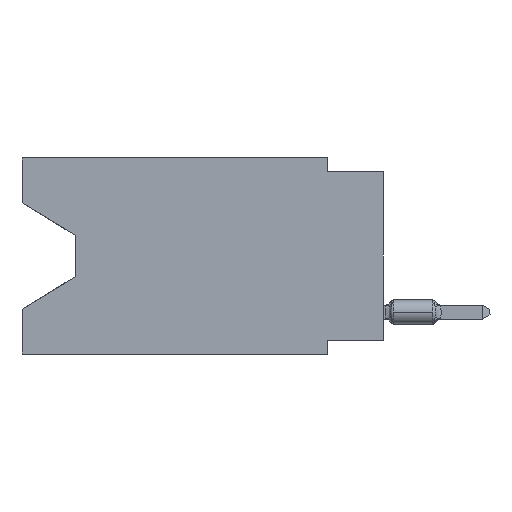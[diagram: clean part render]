
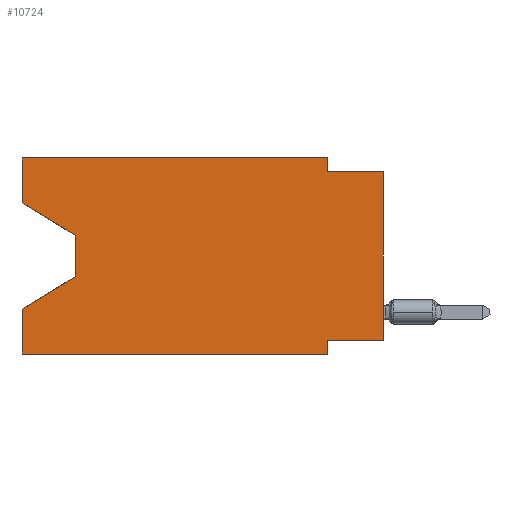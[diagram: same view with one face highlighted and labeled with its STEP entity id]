
A CAD part, left-side view. The second image highlights one B-rep face of the part: STEP entity #10724.
In plain terms, the highlighted planar face has unit normal (-1, 0, 0).
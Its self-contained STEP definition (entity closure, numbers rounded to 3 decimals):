
#278 = VERTEX_POINT ( 'NONE', #18204 ) ;
#285 = FACE_OUTER_BOUND ( 'NONE', #13902, .T. ) ;
#400 = DIRECTION ( 'NONE',  ( 0., 0., 1. ) ) ;
#1129 = CARTESIAN_POINT ( 'NONE',  ( 0., 16.383, 0. ) ) ;
#1442 = EDGE_CURVE ( 'NONE', #11655, #9051, #14736, .T. ) ;
#1532 = VECTOR ( 'NONE', #20490, 1000. ) ;
#1934 = EDGE_CURVE ( 'NONE', #10550, #17345, #22186, .T. ) ;
#1943 = DIRECTION ( 'NONE',  ( 0., 0.855, -0.519 ) ) ;
#2393 = VECTOR ( 'NONE', #400, 1000. ) ;
#2554 = CARTESIAN_POINT ( 'NONE',  ( 0., 16.383, 0. ) ) ;
#2803 = CARTESIAN_POINT ( 'NONE',  ( 0., 16.383, -6.852 ) ) ;
#2872 = VERTEX_POINT ( 'NONE', #6069 ) ;
#3043 = VECTOR ( 'NONE', #10636, 1000. ) ;
#3242 = CARTESIAN_POINT ( 'NONE',  ( 0., 0., -0.635 ) ) ;
#3255 = CARTESIAN_POINT ( 'NONE',  ( 0., 2.54, 0. ) ) ;
#3659 = VECTOR ( 'NONE', #7318, 1000. ) ;
#5485 = DIRECTION ( 'NONE',  ( 0., 0., 1. ) ) ;
#6039 = CARTESIAN_POINT ( 'NONE',  ( 0., 13.97, -3.505 ) ) ;
#6069 = CARTESIAN_POINT ( 'NONE',  ( 0., 2.54, -8.89 ) ) ;
#6123 = LINE ( 'NONE', #11718, #23180 ) ;
#6682 = ORIENTED_EDGE ( 'NONE', *, *, #22969, .T. ) ;
#6735 = EDGE_CURVE ( 'NONE', #21337, #13340, #6123, .T. ) ;
#6909 = DIRECTION ( 'NONE',  ( 0., 0., -1. ) ) ;
#6981 = VECTOR ( 'NONE', #10185, 1000. ) ;
#7128 = DIRECTION ( 'NONE',  ( 0., 0., -1. ) ) ;
#7311 = CARTESIAN_POINT ( 'NONE',  ( 0., 16.383, -8.89 ) ) ;
#7318 = DIRECTION ( 'NONE',  ( 0., 0., -1. ) ) ;
#7470 = ORIENTED_EDGE ( 'NONE', *, *, #23460, .T. ) ;
#7527 = ORIENTED_EDGE ( 'NONE', *, *, #23767, .F. ) ;
#7595 = CARTESIAN_POINT ( 'NONE',  ( 0., 0., -0.635 ) ) ;
#7633 = EDGE_CURVE ( 'NONE', #9051, #19274, #9090, .T. ) ;
#8300 = ORIENTED_EDGE ( 'NONE', *, *, #19170, .F. ) ;
#8531 = LINE ( 'NONE', #1129, #10843 ) ;
#8708 = PLANE ( 'NONE',  #21011 ) ;
#8941 = VERTEX_POINT ( 'NONE', #7311 ) ;
#9051 = VERTEX_POINT ( 'NONE', #17484 ) ;
#9090 = LINE ( 'NONE', #23857, #21678 ) ;
#9175 = LINE ( 'NONE', #3255, #17801 ) ;
#9290 = ORIENTED_EDGE ( 'NONE', *, *, #1442, .T. ) ;
#9470 = LINE ( 'NONE', #11769, #1532 ) ;
#9491 = ORIENTED_EDGE ( 'NONE', *, *, #6735, .T. ) ;
#9552 = EDGE_CURVE ( 'NONE', #278, #13340, #19838, .T. ) ;
#9705 = ORIENTED_EDGE ( 'NONE', *, *, #9552, .F. ) ;
#9934 = LINE ( 'NONE', #11522, #6981 ) ;
#10018 = CARTESIAN_POINT ( 'NONE',  ( 0., 0., -8.255 ) ) ;
#10185 = DIRECTION ( 'NONE',  ( 0., 1., 0. ) ) ;
#10550 = VERTEX_POINT ( 'NONE', #21404 ) ;
#10609 = VERTEX_POINT ( 'NONE', #13924 ) ;
#10636 = DIRECTION ( 'NONE',  ( 0., -1., 0. ) ) ;
#10724 = ADVANCED_FACE ( 'NONE', ( #285 ), #8708, .F. ) ;
#10843 = VECTOR ( 'NONE', #21464, 1000. ) ;
#10988 = ORIENTED_EDGE ( 'NONE', *, *, #11925, .F. ) ;
#11087 = LINE ( 'NONE', #22215, #18148 ) ;
#11203 = CARTESIAN_POINT ( 'NONE',  ( 0., 13.97, -3.505 ) ) ;
#11426 = LINE ( 'NONE', #2554, #2393 ) ;
#11522 = CARTESIAN_POINT ( 'NONE',  ( 0., 0., -8.255 ) ) ;
#11655 = VERTEX_POINT ( 'NONE', #6039 ) ;
#11718 = CARTESIAN_POINT ( 'NONE',  ( 0., 0., 0. ) ) ;
#11769 = CARTESIAN_POINT ( 'NONE',  ( 0., 16.383, -2.038 ) ) ;
#11925 = EDGE_CURVE ( 'NONE', #10609, #278, #9175, .T. ) ;
#12100 = ORIENTED_EDGE ( 'NONE', *, *, #17191, .F. ) ;
#12611 = LINE ( 'NONE', #12855, #16618 ) ;
#12855 = CARTESIAN_POINT ( 'NONE',  ( 0., 2.54, -8.89 ) ) ;
#12881 = CARTESIAN_POINT ( 'NONE',  ( 0., 16.383, 0. ) ) ;
#13073 = CARTESIAN_POINT ( 'NONE',  ( 0., 16.383, 0. ) ) ;
#13144 = CARTESIAN_POINT ( 'NONE',  ( 0., 16.383, 0. ) ) ;
#13340 = VERTEX_POINT ( 'NONE', #7595 ) ;
#13426 = ORIENTED_EDGE ( 'NONE', *, *, #1934, .F. ) ;
#13751 = VECTOR ( 'NONE', #5485, 1000. ) ;
#13902 = EDGE_LOOP ( 'NONE', ( #7470, #9290, #15675, #8300, #6682, #7527, #21201, #9491, #9705, #10988, #12100, #13426 ) ) ;
#13924 = CARTESIAN_POINT ( 'NONE',  ( 0., 2.54, 0. ) ) ;
#14004 = VERTEX_POINT ( 'NONE', #19032 ) ;
#14736 = LINE ( 'NONE', #11203, #3659 ) ;
#15092 = DIRECTION ( 'NONE',  ( 1., 0., 0. ) ) ;
#15675 = ORIENTED_EDGE ( 'NONE', *, *, #7633, .T. ) ;
#15801 = EDGE_CURVE ( 'NONE', #21337, #14004, #9934, .T. ) ;
#16618 = VECTOR ( 'NONE', #6909, 1000. ) ;
#17191 = EDGE_CURVE ( 'NONE', #17345, #10609, #8531, .T. ) ;
#17345 = VERTEX_POINT ( 'NONE', #13073 ) ;
#17484 = CARTESIAN_POINT ( 'NONE',  ( 0., 13.97, -5.385 ) ) ;
#17801 = VECTOR ( 'NONE', #7128, 1000. ) ;
#18148 = VECTOR ( 'NONE', #18468, 1000. ) ;
#18204 = CARTESIAN_POINT ( 'NONE',  ( 0., 2.54, -0.635 ) ) ;
#18468 = DIRECTION ( 'NONE',  ( 0., -1., 0. ) ) ;
#19032 = CARTESIAN_POINT ( 'NONE',  ( 0., 2.54, -8.255 ) ) ;
#19091 = DIRECTION ( 'NONE',  ( 0., 0., 1. ) ) ;
#19170 = EDGE_CURVE ( 'NONE', #8941, #19274, #11426, .T. ) ;
#19274 = VERTEX_POINT ( 'NONE', #2803 ) ;
#19838 = LINE ( 'NONE', #3242, #3043 ) ;
#20490 = DIRECTION ( 'NONE',  ( 0., -0.855, -0.519 ) ) ;
#21011 = AXIS2_PLACEMENT_3D ( 'NONE', #13144, #15092, #21648 ) ;
#21201 = ORIENTED_EDGE ( 'NONE', *, *, #15801, .F. ) ;
#21337 = VERTEX_POINT ( 'NONE', #10018 ) ;
#21404 = CARTESIAN_POINT ( 'NONE',  ( 0., 16.383, -2.038 ) ) ;
#21464 = DIRECTION ( 'NONE',  ( 0., -1., 0. ) ) ;
#21648 = DIRECTION ( 'NONE',  ( 0., 0., -1. ) ) ;
#21678 = VECTOR ( 'NONE', #1943, 1000. ) ;
#22186 = LINE ( 'NONE', #12881, #13751 ) ;
#22215 = CARTESIAN_POINT ( 'NONE',  ( 0., 16.383, -8.89 ) ) ;
#22969 = EDGE_CURVE ( 'NONE', #8941, #2872, #11087, .T. ) ;
#23180 = VECTOR ( 'NONE', #19091, 1000. ) ;
#23460 = EDGE_CURVE ( 'NONE', #10550, #11655, #9470, .T. ) ;
#23767 = EDGE_CURVE ( 'NONE', #14004, #2872, #12611, .T. ) ;
#23857 = CARTESIAN_POINT ( 'NONE',  ( 0., 13.97, -5.385 ) ) ;
